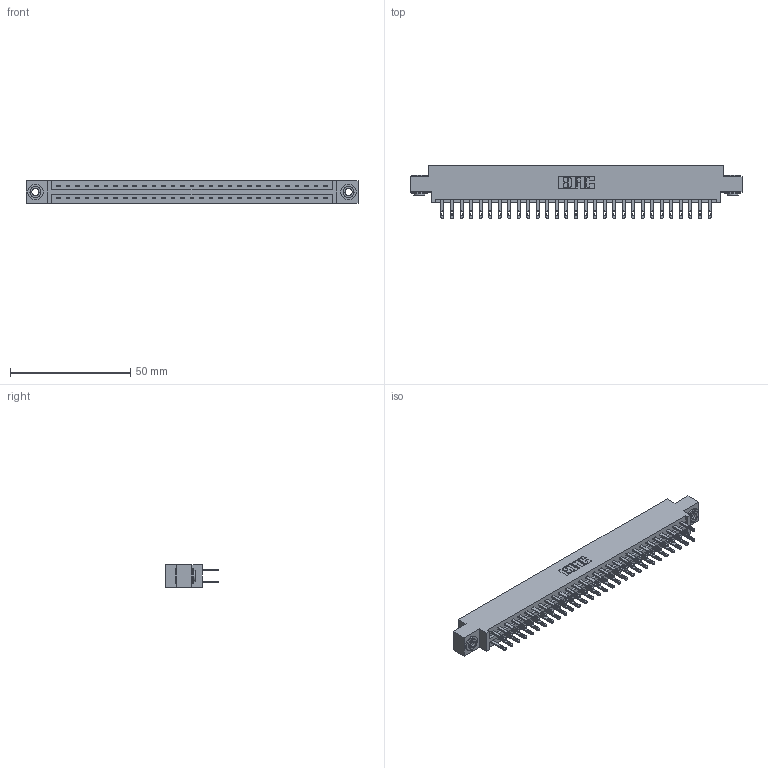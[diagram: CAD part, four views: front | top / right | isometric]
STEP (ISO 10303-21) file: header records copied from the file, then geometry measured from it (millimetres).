
FILE_DESCRIPTION (( 'STEP AP203' ), '1' );
FILE_NAME ('337-058-500-803.STEP', '2018-08-10T04:24:49', ( '' ), ( '' ), 'SwSTEP 2.0', 'SolidWorks 2016', '' );
FILE_SCHEMA (( 'CONFIG_CONTROL_DESIGN' ));
Length unit declared in the file: inch
Products named in the file (4): 337 Part_0.170 Offset - 0.156 Dia-TH; 345-292-001_345-293-100; 345-250-002_345-250-002-102; 337-058-500-803
Assembly tree (61 placements, depth 2):
  337-058-500-803
    337 Part_0.170 Offset - 0.156 Dia-TH
    345-292-001_345-293-100  x58
    345-250-002_345-250-002-102  x2
Bounding box: 137.92 x 21.85 x 9.4 mm (x, y, z)
Volume: 14441.4 mm3; surface area: 17175.5 mm2
Topology: 61 solids, 61 shells, 3056 faces, 9273 edges, 6178 vertices
Faces by surface type: plane 1940, cylinder 1108, cone 8
Entity records: 24878 total; most frequent: CARTESIAN_POINT 4177, ORIENTED_EDGE 4106, DIRECTION 3611, EDGE_CURVE 2053, LINE 1897, VECTOR 1897, VERTEX_POINT 1366, AXIS2_PLACEMENT_3D 857
